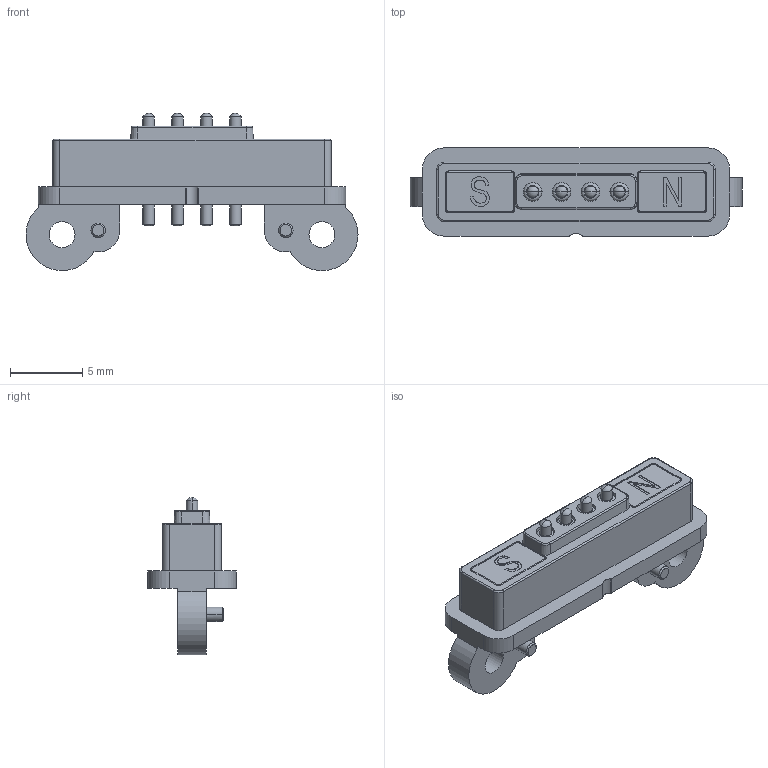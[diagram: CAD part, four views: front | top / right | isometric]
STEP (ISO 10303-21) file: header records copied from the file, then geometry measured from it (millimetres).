
FILE_DESCRIPTION (( 'STEP AP214' ), '1' );
FILE_NAME ('685J0421451124E.STEP', '2023-05-05T19:12:29', ( '' ), ( '' ), 'SwSTEP 2.0', 'SolidWorks 2020', '' );
FILE_SCHEMA (( 'AUTOMOTIVE_DESIGN' ));
Length unit declared in the file: millimetre
Products named in the file (1): 685J0421451124E
Bounding box: 23 x 6.1 x 10.89 mm (x, y, z)
Volume: 480.4 mm3; surface area: 866.1 mm2
Topology: 5 solids, 11 shells, 318 faces, 731 edges, 452 vertices
Faces by surface type: cylinder 132, plane 106, bspline 30, cone 26, torus 16, sphere 8
Entity records: 10769 total; most frequent: CARTESIAN_POINT 2788, DIRECTION 1557, ORIENTED_EDGE 1462, EDGE_CURVE 731, AXIS2_PLACEMENT_3D 593, VERTEX_POINT 452, VECTOR 371, LINE 371
